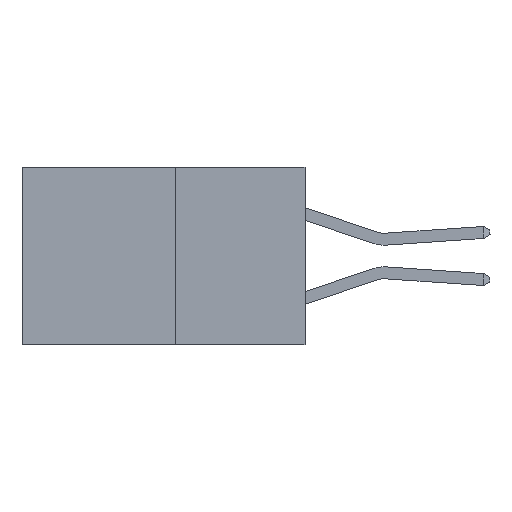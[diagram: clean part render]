
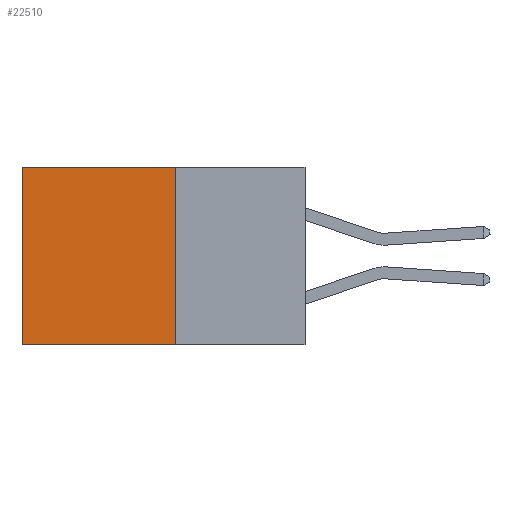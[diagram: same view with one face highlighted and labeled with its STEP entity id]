
A CAD part, left-side view. The second image highlights one B-rep face of the part: STEP entity #22510.
In plain terms, the highlighted planar face has unit normal (-1, 0, 0).
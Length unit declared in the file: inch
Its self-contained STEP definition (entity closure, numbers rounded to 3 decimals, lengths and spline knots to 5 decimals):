
#242 = FACE_OUTER_BOUND ( 'NONE', #31630, .T. ) ;
#1454 = VERTEX_POINT ( 'NONE', #29978 ) ;
#1999 = LINE ( 'NONE', #20561, #29424 ) ;
#3350 = ORIENTED_EDGE ( 'NONE', *, *, #19118, .T. ) ;
#4046 = DIRECTION ( 'NONE',  ( 0., 1., 0. ) ) ;
#4764 = VERTEX_POINT ( 'NONE', #21012 ) ;
#6310 = DIRECTION ( 'NONE',  ( 0., 0., -1. ) ) ;
#6891 = ORIENTED_EDGE ( 'NONE', *, *, #32777, .F. ) ;
#7422 = CARTESIAN_POINT ( 'NONE',  ( 0.277, 0.27, 0. ) ) ;
#8712 = EDGE_CURVE ( 'NONE', #1454, #16544, #1999, .T. ) ;
#9254 = CARTESIAN_POINT ( 'NONE',  ( 0.277, 0.27, -0.37 ) ) ;
#11520 = CARTESIAN_POINT ( 'NONE',  ( 0.277, 0.59, -0.37 ) ) ;
#12742 = LINE ( 'NONE', #9254, #14365 ) ;
#13759 = EDGE_CURVE ( 'NONE', #4764, #27827, #28408, .T. ) ;
#14365 = VECTOR ( 'NONE', #4046, 39.37008 ) ;
#16315 = VECTOR ( 'NONE', #25409, 39.37008 ) ;
#16544 = VERTEX_POINT ( 'NONE', #11520 ) ;
#16549 = PLANE ( 'NONE',  #20644 ) ;
#17240 = CARTESIAN_POINT ( 'NONE',  ( 0.277, 0.27, -0.37 ) ) ;
#19012 = CARTESIAN_POINT ( 'NONE',  ( 0.277, 0.27, -0.37 ) ) ;
#19118 = EDGE_CURVE ( 'NONE', #4764, #1454, #29188, .T. ) ;
#19241 = CARTESIAN_POINT ( 'NONE',  ( 0.277, 0.27, -0.37 ) ) ;
#20195 = ORIENTED_EDGE ( 'NONE', *, *, #13759, .F. ) ;
#20561 = CARTESIAN_POINT ( 'NONE',  ( 0.277, 0.59, -0.37 ) ) ;
#20644 = AXIS2_PLACEMENT_3D ( 'NONE', #19012, #21701, #6310 ) ;
#21012 = CARTESIAN_POINT ( 'NONE',  ( 0.277, 0.27, 0. ) ) ;
#21545 = VECTOR ( 'NONE', #27466, 39.37008 ) ;
#21701 = DIRECTION ( 'NONE',  ( 1., 0., 0. ) ) ;
#22510 = ADVANCED_FACE ( 'NONE', ( #242 ), #16549, .F. ) ;
#23148 = DIRECTION ( 'NONE',  ( 0., 0., -1. ) ) ;
#25409 = DIRECTION ( 'NONE',  ( 0., 1., 0. ) ) ;
#25415 = ORIENTED_EDGE ( 'NONE', *, *, #8712, .T. ) ;
#27466 = DIRECTION ( 'NONE',  ( 0., 0., -1. ) ) ;
#27827 = VERTEX_POINT ( 'NONE', #19241 ) ;
#28408 = LINE ( 'NONE', #17240, #21545 ) ;
#29188 = LINE ( 'NONE', #7422, #16315 ) ;
#29424 = VECTOR ( 'NONE', #23148, 39.37008 ) ;
#29978 = CARTESIAN_POINT ( 'NONE',  ( 0.277, 0.59, 0. ) ) ;
#31630 = EDGE_LOOP ( 'NONE', ( #25415, #6891, #20195, #3350 ) ) ;
#32777 = EDGE_CURVE ( 'NONE', #27827, #16544, #12742, .T. ) ;
